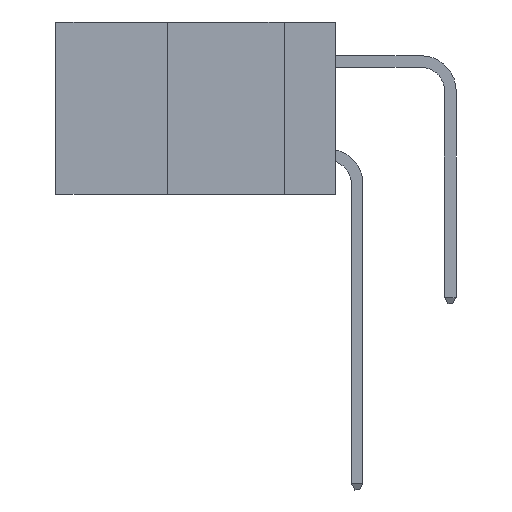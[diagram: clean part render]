
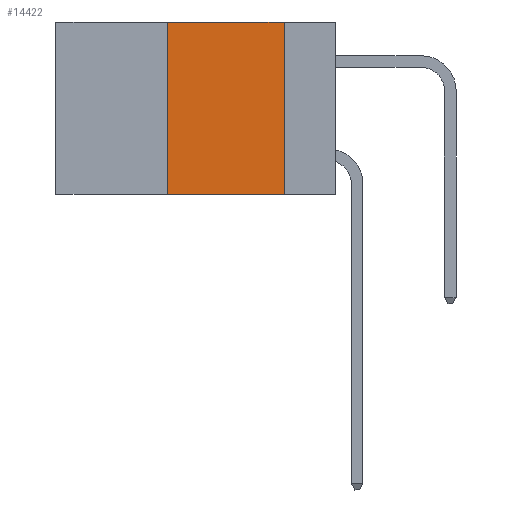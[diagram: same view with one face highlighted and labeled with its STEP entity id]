
A CAD part, left-side view. The second image highlights one B-rep face of the part: STEP entity #14422.
In plain terms, the highlighted planar face has unit normal (-1, 0, 0).
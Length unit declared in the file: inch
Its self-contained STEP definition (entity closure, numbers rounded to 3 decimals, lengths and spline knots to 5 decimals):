
#1092 = CARTESIAN_POINT ( 'NONE',  ( 0., 0.36, 0. ) ) ;
#1267 = ORIENTED_EDGE ( 'NONE', *, *, #9909, .F. ) ;
#3253 = DIRECTION ( 'NONE',  ( 0., -1., 0. ) ) ;
#3332 = DIRECTION ( 'NONE',  ( 0., 0., -1. ) ) ;
#3368 = EDGE_CURVE ( 'NONE', #4466, #10037, #16711, .T. ) ;
#3534 = CARTESIAN_POINT ( 'NONE',  ( 0., 0.11, 0. ) ) ;
#4085 = AXIS2_PLACEMENT_3D ( 'NONE', #8543, #16481, #3332 ) ;
#4466 = VERTEX_POINT ( 'NONE', #5866 ) ;
#5516 = VERTEX_POINT ( 'NONE', #11387 ) ;
#5866 = CARTESIAN_POINT ( 'NONE',  ( 0., 0.36, 0. ) ) ;
#6068 = CARTESIAN_POINT ( 'NONE',  ( 0., 0.6, -0.37 ) ) ;
#6084 = FACE_OUTER_BOUND ( 'NONE', #13661, .T. ) ;
#6117 = LINE ( 'NONE', #6068, #8417 ) ;
#6161 = EDGE_CURVE ( 'NONE', #5516, #4466, #16815, .T. ) ;
#7228 = DIRECTION ( 'NONE',  ( 0., 0., 1. ) ) ;
#7449 = LINE ( 'NONE', #13823, #8052 ) ;
#8052 = VECTOR ( 'NONE', #11223, 39.37008 ) ;
#8417 = VECTOR ( 'NONE', #3253, 39.37008 ) ;
#8543 = CARTESIAN_POINT ( 'NONE',  ( 0., 0.6, 0. ) ) ;
#9776 = ORIENTED_EDGE ( 'NONE', *, *, #3368, .F. ) ;
#9909 = EDGE_CURVE ( 'NONE', #10037, #14682, #7449, .T. ) ;
#10037 = VERTEX_POINT ( 'NONE', #3534 ) ;
#10475 = DIRECTION ( 'NONE',  ( 0., -1., 0. ) ) ;
#10498 = ORIENTED_EDGE ( 'NONE', *, *, #13492, .T. ) ;
#11223 = DIRECTION ( 'NONE',  ( 0., 0., -1. ) ) ;
#11356 = CARTESIAN_POINT ( 'NONE',  ( 0., 0.6, 0. ) ) ;
#11387 = CARTESIAN_POINT ( 'NONE',  ( 0., 0.36, -0.37 ) ) ;
#13492 = EDGE_CURVE ( 'NONE', #5516, #14682, #6117, .T. ) ;
#13661 = EDGE_LOOP ( 'NONE', ( #1267, #9776, #14406, #10498 ) ) ;
#13755 = VECTOR ( 'NONE', #7228, 39.37008 ) ;
#13823 = CARTESIAN_POINT ( 'NONE',  ( 0., 0.11, 0. ) ) ;
#13962 = PLANE ( 'NONE',  #4085 ) ;
#14406 = ORIENTED_EDGE ( 'NONE', *, *, #6161, .F. ) ;
#14412 = CARTESIAN_POINT ( 'NONE',  ( 0., 0.11, -0.37 ) ) ;
#14422 = ADVANCED_FACE ( 'NONE', ( #6084 ), #13962, .F. ) ;
#14682 = VERTEX_POINT ( 'NONE', #14412 ) ;
#15487 = VECTOR ( 'NONE', #10475, 39.37008 ) ;
#16481 = DIRECTION ( 'NONE',  ( 1., 0., 0. ) ) ;
#16711 = LINE ( 'NONE', #11356, #15487 ) ;
#16815 = LINE ( 'NONE', #1092, #13755 ) ;
